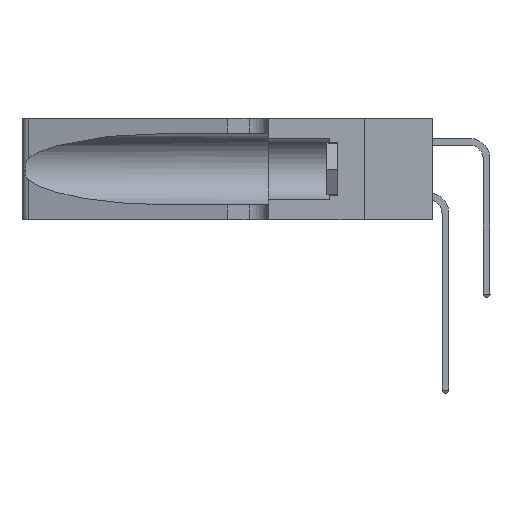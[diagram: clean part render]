
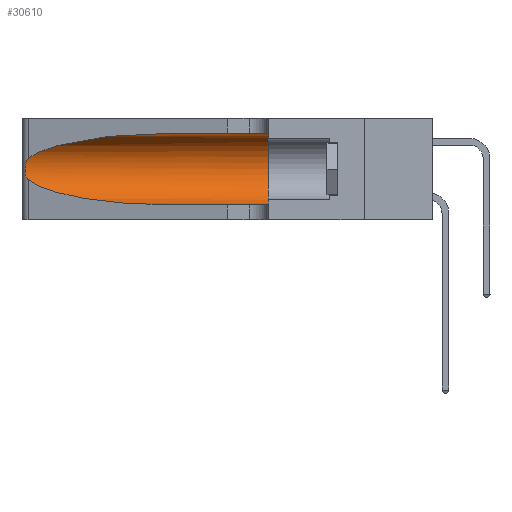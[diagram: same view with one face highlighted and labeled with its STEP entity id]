
A CAD part, left-side view. The second image highlights one B-rep face of the part: STEP entity #30610.
In plain terms, the highlighted cylindrical face has radius 3.308 mm (diameter 6.617 mm), a partial arc.
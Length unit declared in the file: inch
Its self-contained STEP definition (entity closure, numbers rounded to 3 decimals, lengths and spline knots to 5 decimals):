
#575 = CARTESIAN_POINT ( 'NONE',  ( 0.25789, 1.23486, 0.15765 ) ) ;
#2379 = B_SPLINE_CURVE_WITH_KNOTS ( 'NONE', 3,
 ( #20645, #26450, #35484, #15130, #12350, #3370, #23956, #23834, #9704, #9191, #575, #18129, #20774, #35356 ),
 .UNSPECIFIED., .F., .F.,
 ( 4, 2, 2, 2, 2, 2, 4 ),
 ( 0., 0.00027, 0.00053, 0.00107, 0.0016, 0.00187, 0.00214 ),
 .UNSPECIFIED. ) ;
#2667 = ORIENTED_EDGE ( 'NONE', *, *, #12339, .T. ) ;
#2720 = VECTOR ( 'NONE', #6337, 39.37008 ) ;
#3370 = CARTESIAN_POINT ( 'NONE',  ( 0.26018, 1.23835, 0.19895 ) ) ;
#4888 = AXIS2_PLACEMENT_3D ( 'NONE', #17618, #29510, #26207 ) ;
#5053 = CARTESIAN_POINT ( 'NONE',  ( 0.18966, 0.96281, 0.31525 ) ) ;
#5350 = VERTEX_POINT ( 'NONE', #21650 ) ;
#5353 = ORIENTED_EDGE ( 'NONE', *, *, #23826, .F. ) ;
#5863 = CARTESIAN_POINT ( 'NONE',  ( 0.1305, 1.61858, 0.31525 ) ) ;
#5977 = AXIS2_PLACEMENT_3D ( 'NONE', #13608, #33614, #10350 ) ;
#6210 = VERTEX_POINT ( 'NONE', #13522 ) ;
#6337 = DIRECTION ( 'NONE',  ( 0., -1., 0. ) ) ;
#7618 = VERTEX_POINT ( 'NONE', #33124 ) ;
#7700 = CARTESIAN_POINT ( 'NONE',  ( 0.25487, 1.22718, 0.22369 ) ) ;
#7847 = CARTESIAN_POINT ( 'NONE',  ( 0.1305, 0.35, 0.05475 ) ) ;
#8308 = ORIENTED_EDGE ( 'NONE', *, *, #26225, .F. ) ;
#9052 =( BOUNDED_CURVE ( )  B_SPLINE_CURVE ( 3, ( #14294, #11743, #9064, #17186 ),
 .UNSPECIFIED., .F., .F. ) 
 B_SPLINE_CURVE_WITH_KNOTS ( ( 4, 4 ),
 ( 3.44316, 4.71239 ),
 .UNSPECIFIED. ) 
 CURVE ( )  GEOMETRIC_REPRESENTATION_ITEM ( )  RATIONAL_B_SPLINE_CURVE ( ( 1., 0.87, 0.87, 1. ) ) 
 REPRESENTATION_ITEM ( '' )  );
#9064 = CARTESIAN_POINT ( 'NONE',  ( 0.18966, 0.96281, 0.05475 ) ) ;
#9191 = CARTESIAN_POINT ( 'NONE',  ( 0.25856, 1.23593, 0.16098 ) ) ;
#9704 = CARTESIAN_POINT ( 'NONE',  ( 0.26017, 1.23833, 0.17102 ) ) ;
#10350 = DIRECTION ( 'NONE',  ( 0., 0., -1. ) ) ;
#11711 = ORIENTED_EDGE ( 'NONE', *, *, #14111, .T. ) ;
#11743 = CARTESIAN_POINT ( 'NONE',  ( 0.2373, 1.15595, 0.08982 ) ) ;
#12339 = EDGE_CURVE ( 'NONE', #7618, #22680, #31211, .T. ) ;
#12349 = CIRCLE ( 'NONE', #4888, 0.13025 ) ;
#12350 = CARTESIAN_POINT ( 'NONE',  ( 0.25854, 1.2359, 0.20912 ) ) ;
#12997 = VECTOR ( 'NONE', #19866, 39.37008 ) ;
#13522 = CARTESIAN_POINT ( 'NONE',  ( 0.25487, 1.22718, 0.14631 ) ) ;
#13608 = CARTESIAN_POINT ( 'NONE',  ( 0.1305, 1.61858, 0.185 ) ) ;
#14111 = EDGE_CURVE ( 'NONE', #5350, #6210, #2379, .T. ) ;
#14294 = CARTESIAN_POINT ( 'NONE',  ( 0.25487, 1.22718, 0.14631 ) ) ;
#15130 = CARTESIAN_POINT ( 'NONE',  ( 0.25787, 1.23484, 0.2124 ) ) ;
#15215 = ORIENTED_EDGE ( 'NONE', *, *, #28388, .T. ) ;
#17186 = CARTESIAN_POINT ( 'NONE',  ( 0.1305, 0.72297, 0.05475 ) ) ;
#17618 = CARTESIAN_POINT ( 'NONE',  ( 0.1305, 0.35, 0.185 ) ) ;
#18063 = CARTESIAN_POINT ( 'NONE',  ( 0.1305, 1.61858, 0.05475 ) ) ;
#18129 = CARTESIAN_POINT ( 'NONE',  ( 0.25639, 1.23186, 0.15144 ) ) ;
#18732 = CARTESIAN_POINT ( 'NONE',  ( 0.1305, 0.72297, 0.31525 ) ) ;
#19866 = DIRECTION ( 'NONE',  ( 0., -1., 0. ) ) ;
#20645 = CARTESIAN_POINT ( 'NONE',  ( 0.25487, 1.22718, 0.22369 ) ) ;
#20774 = CARTESIAN_POINT ( 'NONE',  ( 0.25555, 1.22993, 0.14849 ) ) ;
#20837 =( BOUNDED_CURVE ( )  B_SPLINE_CURVE ( 3, ( #36641, #5053, #27652, #7700 ),
 .UNSPECIFIED., .F., .T. ) 
 B_SPLINE_CURVE_WITH_KNOTS ( ( 4, 4 ),
 ( 1.5708, 2.84003 ),
 .UNSPECIFIED. ) 
 CURVE ( )  GEOMETRIC_REPRESENTATION_ITEM ( )  RATIONAL_B_SPLINE_CURVE ( ( 1., 0.87, 0.87, 1. ) ) 
 REPRESENTATION_ITEM ( '' )  );
#21650 = CARTESIAN_POINT ( 'NONE',  ( 0.25487, 1.22718, 0.22369 ) ) ;
#22009 = LINE ( 'NONE', #5863, #12997 ) ;
#22680 = VERTEX_POINT ( 'NONE', #7847 ) ;
#23103 = FACE_OUTER_BOUND ( 'NONE', #34539, .T. ) ;
#23826 = EDGE_CURVE ( 'NONE', #24713, #22680, #12349, .T. ) ;
#23834 = CARTESIAN_POINT ( 'NONE',  ( 0.26075, 1.23896, 0.178 ) ) ;
#23956 = CARTESIAN_POINT ( 'NONE',  ( 0.26075, 1.23896, 0.19203 ) ) ;
#24713 = VERTEX_POINT ( 'NONE', #24927 ) ;
#24927 = CARTESIAN_POINT ( 'NONE',  ( 0.1305, 0.35, 0.31525 ) ) ;
#26207 = DIRECTION ( 'NONE',  ( 0., 0., 1. ) ) ;
#26225 = EDGE_CURVE ( 'NONE', #31016, #24713, #22009, .T. ) ;
#26450 = CARTESIAN_POINT ( 'NONE',  ( 0.25555, 1.22994, 0.2215 ) ) ;
#27652 = CARTESIAN_POINT ( 'NONE',  ( 0.2373, 1.15595, 0.28018 ) ) ;
#28388 = EDGE_CURVE ( 'NONE', #6210, #7618, #9052, .T. ) ;
#29510 = DIRECTION ( 'NONE',  ( 0., 1., 0. ) ) ;
#30610 = ADVANCED_FACE ( 'NONE', ( #23103 ), #35746, .F. ) ;
#31016 = VERTEX_POINT ( 'NONE', #18732 ) ;
#31211 = LINE ( 'NONE', #18063, #2720 ) ;
#33124 = CARTESIAN_POINT ( 'NONE',  ( 0.1305, 0.72297, 0.05475 ) ) ;
#33614 = DIRECTION ( 'NONE',  ( 0., -1., 0. ) ) ;
#34539 = EDGE_LOOP ( 'NONE', ( #36787, #11711, #15215, #2667, #5353, #8308 ) ) ;
#35356 = CARTESIAN_POINT ( 'NONE',  ( 0.25487, 1.22718, 0.14631 ) ) ;
#35484 = CARTESIAN_POINT ( 'NONE',  ( 0.25639, 1.23184, 0.21858 ) ) ;
#35746 = CYLINDRICAL_SURFACE ( 'NONE', #5977, 0.13025 ) ;
#35753 = EDGE_CURVE ( 'NONE', #31016, #5350, #20837, .T. ) ;
#36641 = CARTESIAN_POINT ( 'NONE',  ( 0.1305, 0.72297, 0.31525 ) ) ;
#36787 = ORIENTED_EDGE ( 'NONE', *, *, #35753, .T. ) ;
